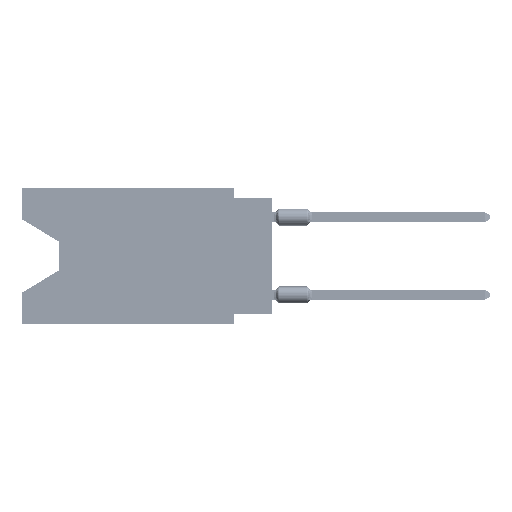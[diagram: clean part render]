
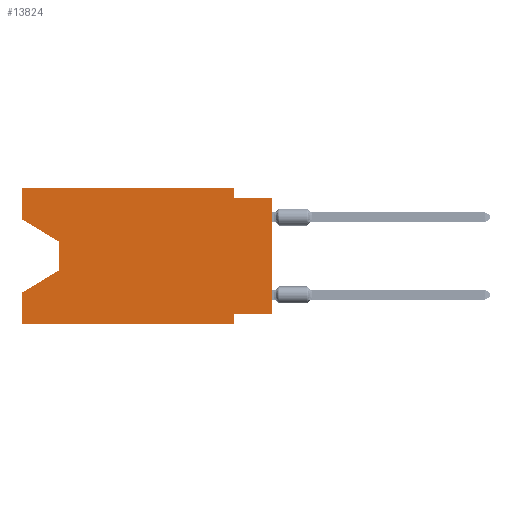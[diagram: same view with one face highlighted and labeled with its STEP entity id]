
A CAD part, left-side view. The second image highlights one B-rep face of the part: STEP entity #13824.
In plain terms, the highlighted planar face has unit normal (-1, 0, 0).
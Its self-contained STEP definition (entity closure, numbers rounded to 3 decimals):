
#172 = CARTESIAN_POINT ( 'NONE',  ( 0., 0., -8.255 ) ) ;
#283 = CARTESIAN_POINT ( 'NONE',  ( 0., 2.54, -0.635 ) ) ;
#469 = CARTESIAN_POINT ( 'NONE',  ( 0., 16.383, -8.89 ) ) ;
#1390 = EDGE_CURVE ( 'NONE', #55712, #13168, #36228, .T. ) ;
#1412 = ORIENTED_EDGE ( 'NONE', *, *, #26683, .F. ) ;
#1660 = CARTESIAN_POINT ( 'NONE',  ( 0., 13.97, -3.505 ) ) ;
#1744 = EDGE_CURVE ( 'NONE', #13168, #80878, #64030, .T. ) ;
#1833 = EDGE_CURVE ( 'NONE', #51162, #73422, #57000, .T. ) ;
#4094 = ORIENTED_EDGE ( 'NONE', *, *, #43812, .F. ) ;
#4446 = VERTEX_POINT ( 'NONE', #15852 ) ;
#5158 = EDGE_CURVE ( 'NONE', #26688, #80878, #33712, .T. ) ;
#5625 = LINE ( 'NONE', #44016, #62508 ) ;
#5696 = VECTOR ( 'NONE', #30079, 1000. ) ;
#6039 = DIRECTION ( 'NONE',  ( 0., -0.855, -0.519 ) ) ;
#7589 = VERTEX_POINT ( 'NONE', #10141 ) ;
#8283 = EDGE_LOOP ( 'NONE', ( #37836, #69846, #13888, #80069, #64468, #1412, #29834, #34328, #11960, #58972, #21492, #4094 ) ) ;
#9991 = PLANE ( 'NONE',  #73098 ) ;
#10141 = CARTESIAN_POINT ( 'NONE',  ( 0., 2.54, -8.255 ) ) ;
#10804 = FACE_OUTER_BOUND ( 'NONE', #8283, .T. ) ;
#11960 = ORIENTED_EDGE ( 'NONE', *, *, #1744, .F. ) ;
#12278 = CARTESIAN_POINT ( 'NONE',  ( 0., 2.54, 0. ) ) ;
#12448 = EDGE_CURVE ( 'NONE', #26688, #7589, #17535, .T. ) ;
#13168 = VERTEX_POINT ( 'NONE', #283 ) ;
#13824 = ADVANCED_FACE ( 'NONE', ( #10804 ), #9991, .F. ) ;
#13888 = ORIENTED_EDGE ( 'NONE', *, *, #77858, .T. ) ;
#14004 = VERTEX_POINT ( 'NONE', #1660 ) ;
#14875 = VECTOR ( 'NONE', #77060, 1000. ) ;
#15852 = CARTESIAN_POINT ( 'NONE',  ( 0., 16.383, -2.038 ) ) ;
#16100 = DIRECTION ( 'NONE',  ( 0., 0.855, -0.519 ) ) ;
#17535 = LINE ( 'NONE', #172, #65031 ) ;
#17702 = CARTESIAN_POINT ( 'NONE',  ( 0., 0., -8.255 ) ) ;
#19486 = VECTOR ( 'NONE', #62626, 1000. ) ;
#21492 = ORIENTED_EDGE ( 'NONE', *, *, #43867, .F. ) ;
#21554 = DIRECTION ( 'NONE',  ( 0., 0., -1. ) ) ;
#22952 = EDGE_CURVE ( 'NONE', #51162, #63446, #74927, .T. ) ;
#23571 = VECTOR ( 'NONE', #37191, 1000. ) ;
#23737 = DIRECTION ( 'NONE',  ( 0., 1., 0. ) ) ;
#25642 = DIRECTION ( 'NONE',  ( 0., -1., 0. ) ) ;
#26683 = EDGE_CURVE ( 'NONE', #7589, #73422, #74648, .T. ) ;
#26688 = VERTEX_POINT ( 'NONE', #17702 ) ;
#27251 = LINE ( 'NONE', #46635, #40217 ) ;
#29115 = CARTESIAN_POINT ( 'NONE',  ( 0., 16.383, 0. ) ) ;
#29480 = VECTOR ( 'NONE', #68301, 1000. ) ;
#29834 = ORIENTED_EDGE ( 'NONE', *, *, #12448, .F. ) ;
#30079 = DIRECTION ( 'NONE',  ( 0., 0., -1. ) ) ;
#32101 = VECTOR ( 'NONE', #57101, 1000. ) ;
#33256 = VECTOR ( 'NONE', #43151, 1000. ) ;
#33712 = LINE ( 'NONE', #59710, #14875 ) ;
#34328 = ORIENTED_EDGE ( 'NONE', *, *, #5158, .T. ) ;
#36066 = EDGE_CURVE ( 'NONE', #14004, #81442, #61850, .T. ) ;
#36088 = CARTESIAN_POINT ( 'NONE',  ( 0., 2.54, 0. ) ) ;
#36228 = LINE ( 'NONE', #12278, #19486 ) ;
#37191 = DIRECTION ( 'NONE',  ( 0., -1., 0. ) ) ;
#37836 = ORIENTED_EDGE ( 'NONE', *, *, #56493, .T. ) ;
#38106 = LINE ( 'NONE', #69514, #32101 ) ;
#40217 = VECTOR ( 'NONE', #16100, 1000. ) ;
#43101 = LINE ( 'NONE', #43498, #29480 ) ;
#43151 = DIRECTION ( 'NONE',  ( 0., 0., 1. ) ) ;
#43263 = CARTESIAN_POINT ( 'NONE',  ( 0., 13.97, -3.505 ) ) ;
#43498 = CARTESIAN_POINT ( 'NONE',  ( 0., 16.383, 0. ) ) ;
#43733 = VERTEX_POINT ( 'NONE', #29115 ) ;
#43812 = EDGE_CURVE ( 'NONE', #4446, #43733, #38106, .T. ) ;
#43867 = EDGE_CURVE ( 'NONE', #43733, #55712, #43101, .T. ) ;
#44016 = CARTESIAN_POINT ( 'NONE',  ( 0., 16.383, -2.038 ) ) ;
#44220 = CARTESIAN_POINT ( 'NONE',  ( 0., 0., -0.635 ) ) ;
#46635 = CARTESIAN_POINT ( 'NONE',  ( 0., 13.97, -5.385 ) ) ;
#48664 = CARTESIAN_POINT ( 'NONE',  ( 0., 2.54, -8.89 ) ) ;
#49881 = VECTOR ( 'NONE', #25642, 1000. ) ;
#51162 = VERTEX_POINT ( 'NONE', #63458 ) ;
#53455 = CARTESIAN_POINT ( 'NONE',  ( 0., 16.383, -6.852 ) ) ;
#54544 = CARTESIAN_POINT ( 'NONE',  ( 0., 16.383, 0. ) ) ;
#55546 = CARTESIAN_POINT ( 'NONE',  ( 0., 16.383, 0. ) ) ;
#55712 = VERTEX_POINT ( 'NONE', #36088 ) ;
#56493 = EDGE_CURVE ( 'NONE', #4446, #14004, #5625, .T. ) ;
#57000 = LINE ( 'NONE', #469, #49881 ) ;
#57101 = DIRECTION ( 'NONE',  ( 0., 0., 1. ) ) ;
#58972 = ORIENTED_EDGE ( 'NONE', *, *, #1390, .F. ) ;
#59710 = CARTESIAN_POINT ( 'NONE',  ( 0., 0., 0. ) ) ;
#60295 = CARTESIAN_POINT ( 'NONE',  ( 0., 13.97, -5.385 ) ) ;
#61850 = LINE ( 'NONE', #43263, #5696 ) ;
#62508 = VECTOR ( 'NONE', #6039, 1000. ) ;
#62626 = DIRECTION ( 'NONE',  ( 0., 0., -1. ) ) ;
#63446 = VERTEX_POINT ( 'NONE', #53455 ) ;
#63458 = CARTESIAN_POINT ( 'NONE',  ( 0., 16.383, -8.89 ) ) ;
#64030 = LINE ( 'NONE', #44220, #23571 ) ;
#64468 = ORIENTED_EDGE ( 'NONE', *, *, #1833, .T. ) ;
#65031 = VECTOR ( 'NONE', #23737, 1000. ) ;
#67666 = DIRECTION ( 'NONE',  ( 0., 0., -1. ) ) ;
#67894 = VECTOR ( 'NONE', #67666, 1000. ) ;
#68301 = DIRECTION ( 'NONE',  ( 0., -1., 0. ) ) ;
#69514 = CARTESIAN_POINT ( 'NONE',  ( 0., 16.383, 0. ) ) ;
#69846 = ORIENTED_EDGE ( 'NONE', *, *, #36066, .T. ) ;
#73098 = AXIS2_PLACEMENT_3D ( 'NONE', #54544, #78095, #21554 ) ;
#73422 = VERTEX_POINT ( 'NONE', #76317 ) ;
#74648 = LINE ( 'NONE', #48664, #67894 ) ;
#74927 = LINE ( 'NONE', #55546, #33256 ) ;
#76317 = CARTESIAN_POINT ( 'NONE',  ( 0., 2.54, -8.89 ) ) ;
#77060 = DIRECTION ( 'NONE',  ( 0., 0., 1. ) ) ;
#77858 = EDGE_CURVE ( 'NONE', #81442, #63446, #27251, .T. ) ;
#78095 = DIRECTION ( 'NONE',  ( 1., 0., 0. ) ) ;
#78842 = CARTESIAN_POINT ( 'NONE',  ( 0., 0., -0.635 ) ) ;
#80069 = ORIENTED_EDGE ( 'NONE', *, *, #22952, .F. ) ;
#80878 = VERTEX_POINT ( 'NONE', #78842 ) ;
#81442 = VERTEX_POINT ( 'NONE', #60295 ) ;
